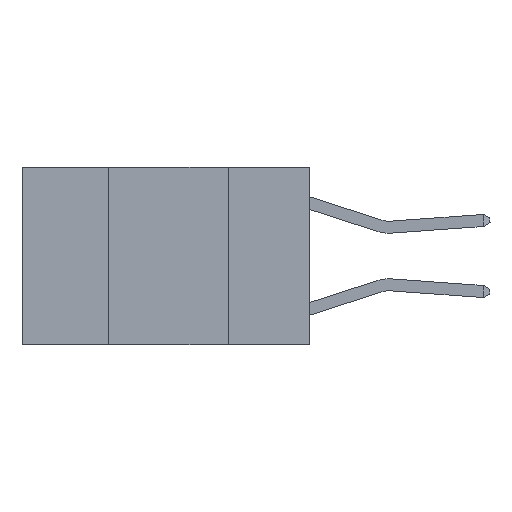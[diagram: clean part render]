
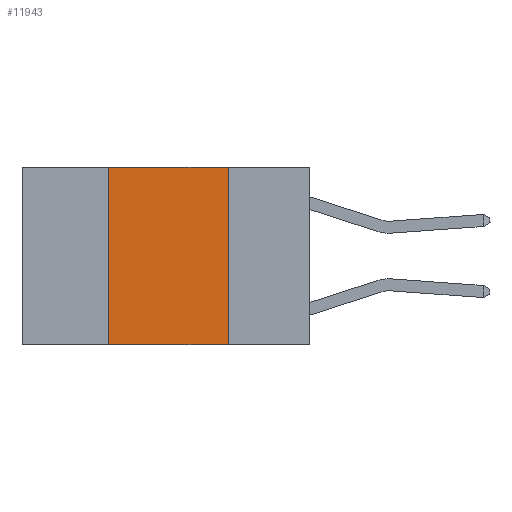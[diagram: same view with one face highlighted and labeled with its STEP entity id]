
A CAD part, left-side view. The second image highlights one B-rep face of the part: STEP entity #11943.
In plain terms, the highlighted planar face has unit normal (-1, 0, 0).
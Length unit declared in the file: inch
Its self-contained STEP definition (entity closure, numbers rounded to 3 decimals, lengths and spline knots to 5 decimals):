
#395 = CARTESIAN_POINT ( 'NONE',  ( 0., 0.6, 0. ) ) ;
#1290 = VECTOR ( 'NONE', #7182, 39.37008 ) ;
#1953 = LINE ( 'NONE', #2067, #10842 ) ;
#2067 = CARTESIAN_POINT ( 'NONE',  ( 0., 0.6, 0. ) ) ;
#2725 = ORIENTED_EDGE ( 'NONE', *, *, #4462, .T. ) ;
#3193 = VERTEX_POINT ( 'NONE', #10384 ) ;
#3964 = ORIENTED_EDGE ( 'NONE', *, *, #15155, .F. ) ;
#4462 = EDGE_CURVE ( 'NONE', #9352, #3193, #13930, .T. ) ;
#4468 = DIRECTION ( 'NONE',  ( 0., 0., -1. ) ) ;
#4500 = VERTEX_POINT ( 'NONE', #9247 ) ;
#5511 = DIRECTION ( 'NONE',  ( 0., -1., 0. ) ) ;
#5580 = EDGE_CURVE ( 'NONE', #4500, #3193, #8113, .T. ) ;
#5641 = CARTESIAN_POINT ( 'NONE',  ( 0., 0.42, 0. ) ) ;
#5657 = PLANE ( 'NONE',  #8972 ) ;
#7182 = DIRECTION ( 'NONE',  ( 0., 0., -1. ) ) ;
#7752 = ORIENTED_EDGE ( 'NONE', *, *, #16248, .F. ) ;
#8113 = LINE ( 'NONE', #15735, #1290 ) ;
#8433 = DIRECTION ( 'NONE',  ( 0., 0., 1. ) ) ;
#8703 = LINE ( 'NONE', #15737, #14814 ) ;
#8972 = AXIS2_PLACEMENT_3D ( 'NONE', #395, #11837, #4468 ) ;
#9247 = CARTESIAN_POINT ( 'NONE',  ( 0., 0.17, 0. ) ) ;
#9352 = VERTEX_POINT ( 'NONE', #13987 ) ;
#10181 = EDGE_LOOP ( 'NONE', ( #14155, #3964, #7752, #2725 ) ) ;
#10384 = CARTESIAN_POINT ( 'NONE',  ( 0., 0.17, -0.37 ) ) ;
#10842 = VECTOR ( 'NONE', #10894, 39.37008 ) ;
#10894 = DIRECTION ( 'NONE',  ( 0., -1., 0. ) ) ;
#11837 = DIRECTION ( 'NONE',  ( 1., 0., 0. ) ) ;
#11943 = ADVANCED_FACE ( 'NONE', ( #13147 ), #5657, .F. ) ;
#12860 = CARTESIAN_POINT ( 'NONE',  ( 0., 0.6, -0.37 ) ) ;
#13147 = FACE_OUTER_BOUND ( 'NONE', #10181, .T. ) ;
#13930 = LINE ( 'NONE', #12860, #14308 ) ;
#13987 = CARTESIAN_POINT ( 'NONE',  ( 0., 0.42, -0.37 ) ) ;
#14155 = ORIENTED_EDGE ( 'NONE', *, *, #5580, .F. ) ;
#14308 = VECTOR ( 'NONE', #5511, 39.37008 ) ;
#14814 = VECTOR ( 'NONE', #8433, 39.37008 ) ;
#15155 = EDGE_CURVE ( 'NONE', #16174, #4500, #1953, .T. ) ;
#15735 = CARTESIAN_POINT ( 'NONE',  ( 0., 0.17, 0. ) ) ;
#15737 = CARTESIAN_POINT ( 'NONE',  ( 0., 0.42, 0. ) ) ;
#16174 = VERTEX_POINT ( 'NONE', #5641 ) ;
#16248 = EDGE_CURVE ( 'NONE', #9352, #16174, #8703, .T. ) ;
